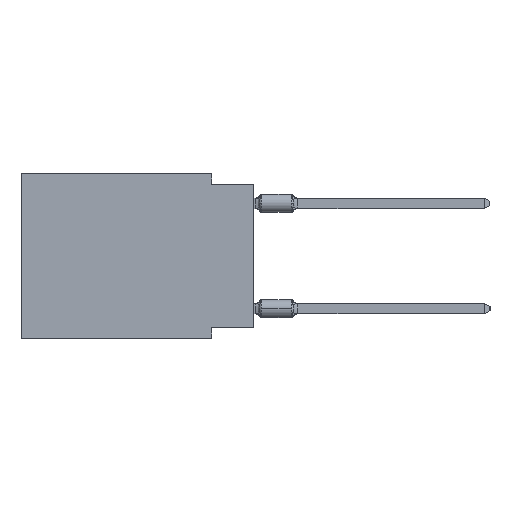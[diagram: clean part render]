
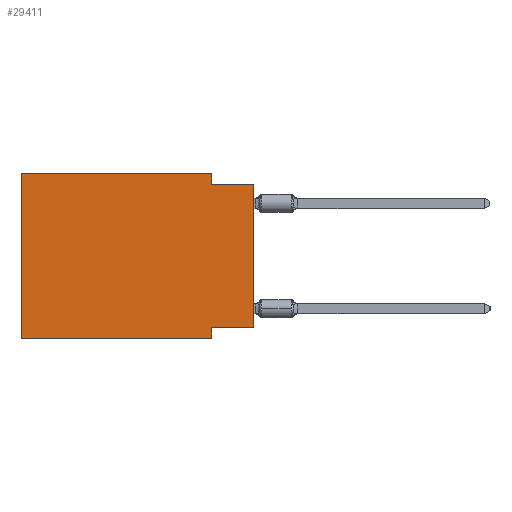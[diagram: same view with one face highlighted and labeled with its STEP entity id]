
A CAD part, left-side view. The second image highlights one B-rep face of the part: STEP entity #29411.
In plain terms, the highlighted planar face has unit normal (-1, 0, 0).
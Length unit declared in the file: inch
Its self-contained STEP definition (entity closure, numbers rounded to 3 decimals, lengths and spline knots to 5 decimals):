
#91 = CARTESIAN_POINT ( 'NONE',  ( 0., 0.1, -0.365 ) ) ;
#154 = ORIENTED_EDGE ( 'NONE', *, *, #16159, .F. ) ;
#680 = CARTESIAN_POINT ( 'NONE',  ( 0., 0.55, 0. ) ) ;
#1687 = EDGE_CURVE ( 'NONE', #15948, #11077, #4665, .T. ) ;
#2459 = EDGE_CURVE ( 'NONE', #29000, #2518, #9080, .T. ) ;
#2518 = VERTEX_POINT ( 'NONE', #11415 ) ;
#3377 = CARTESIAN_POINT ( 'NONE',  ( 0., 0., -0.025 ) ) ;
#4308 = DIRECTION ( 'NONE',  ( 0., 0., -1. ) ) ;
#4665 = LINE ( 'NONE', #29237, #20906 ) ;
#4811 = ORIENTED_EDGE ( 'NONE', *, *, #1687, .T. ) ;
#6917 = VERTEX_POINT ( 'NONE', #23488 ) ;
#7580 = EDGE_CURVE ( 'NONE', #6917, #11077, #14457, .T. ) ;
#8152 = CARTESIAN_POINT ( 'NONE',  ( 0., 0.55, -0.39 ) ) ;
#9080 = LINE ( 'NONE', #680, #9454 ) ;
#9454 = VECTOR ( 'NONE', #25058, 39.37008 ) ;
#10279 = LINE ( 'NONE', #32325, #34799 ) ;
#11077 = VERTEX_POINT ( 'NONE', #31415 ) ;
#11321 = CARTESIAN_POINT ( 'NONE',  ( 0., 0., -0.365 ) ) ;
#11415 = CARTESIAN_POINT ( 'NONE',  ( 0., 0.55, 0. ) ) ;
#11585 = DIRECTION ( 'NONE',  ( 0., -1., 0. ) ) ;
#12739 = DIRECTION ( 'NONE',  ( 0., -1., 0. ) ) ;
#14457 = LINE ( 'NONE', #3377, #26377 ) ;
#14551 = CARTESIAN_POINT ( 'NONE',  ( 0., 0.1, -0.39 ) ) ;
#14753 = CARTESIAN_POINT ( 'NONE',  ( 0., 0.1, 0. ) ) ;
#15461 = EDGE_LOOP ( 'NONE', ( #4811, #27877, #154, #27542, #32997, #31317, #32858, #18688 ) ) ;
#15916 = PLANE ( 'NONE',  #20874 ) ;
#15948 = VERTEX_POINT ( 'NONE', #11321 ) ;
#16159 = EDGE_CURVE ( 'NONE', #31626, #6917, #21309, .T. ) ;
#18160 = CARTESIAN_POINT ( 'NONE',  ( 0., 0.55, -0.39 ) ) ;
#18423 = CARTESIAN_POINT ( 'NONE',  ( 0., 0.55, 0. ) ) ;
#18688 = ORIENTED_EDGE ( 'NONE', *, *, #34823, .F. ) ;
#19564 = EDGE_CURVE ( 'NONE', #29000, #26965, #24652, .T. ) ;
#20874 = AXIS2_PLACEMENT_3D ( 'NONE', #18423, #32076, #26177 ) ;
#20906 = VECTOR ( 'NONE', #34400, 39.37008 ) ;
#21309 = LINE ( 'NONE', #24744, #24211 ) ;
#21341 = LINE ( 'NONE', #21524, #30216 ) ;
#21524 = CARTESIAN_POINT ( 'NONE',  ( 0., 0.55, 0. ) ) ;
#22774 = LINE ( 'NONE', #28706, #32458 ) ;
#22992 = EDGE_CURVE ( 'NONE', #2518, #31626, #21341, .T. ) ;
#23488 = CARTESIAN_POINT ( 'NONE',  ( 0., 0.1, -0.025 ) ) ;
#24211 = VECTOR ( 'NONE', #35107, 39.37008 ) ;
#24272 = DIRECTION ( 'NONE',  ( 0., 1., 0. ) ) ;
#24466 = DIRECTION ( 'NONE',  ( 0., -1., 0. ) ) ;
#24531 = EDGE_CURVE ( 'NONE', #26828, #26965, #22774, .T. ) ;
#24652 = LINE ( 'NONE', #8152, #33983 ) ;
#24744 = CARTESIAN_POINT ( 'NONE',  ( 0., 0.1, 0. ) ) ;
#25058 = DIRECTION ( 'NONE',  ( 0., 0., 1. ) ) ;
#26177 = DIRECTION ( 'NONE',  ( 0., 0., -1. ) ) ;
#26377 = VECTOR ( 'NONE', #11585, 39.37008 ) ;
#26828 = VERTEX_POINT ( 'NONE', #91 ) ;
#26965 = VERTEX_POINT ( 'NONE', #14551 ) ;
#27542 = ORIENTED_EDGE ( 'NONE', *, *, #22992, .F. ) ;
#27877 = ORIENTED_EDGE ( 'NONE', *, *, #7580, .F. ) ;
#28706 = CARTESIAN_POINT ( 'NONE',  ( 0., 0.1, -0.39 ) ) ;
#29000 = VERTEX_POINT ( 'NONE', #18160 ) ;
#29237 = CARTESIAN_POINT ( 'NONE',  ( 0., 0., 0. ) ) ;
#29393 = FACE_OUTER_BOUND ( 'NONE', #15461, .T. ) ;
#29411 = ADVANCED_FACE ( 'NONE', ( #29393 ), #15916, .F. ) ;
#30216 = VECTOR ( 'NONE', #12739, 39.37008 ) ;
#31317 = ORIENTED_EDGE ( 'NONE', *, *, #19564, .T. ) ;
#31415 = CARTESIAN_POINT ( 'NONE',  ( 0., 0., -0.025 ) ) ;
#31626 = VERTEX_POINT ( 'NONE', #14753 ) ;
#32076 = DIRECTION ( 'NONE',  ( 1., 0., 0. ) ) ;
#32325 = CARTESIAN_POINT ( 'NONE',  ( 0., 0., -0.365 ) ) ;
#32458 = VECTOR ( 'NONE', #4308, 39.37008 ) ;
#32858 = ORIENTED_EDGE ( 'NONE', *, *, #24531, .F. ) ;
#32997 = ORIENTED_EDGE ( 'NONE', *, *, #2459, .F. ) ;
#33983 = VECTOR ( 'NONE', #24466, 39.37008 ) ;
#34400 = DIRECTION ( 'NONE',  ( 0., 0., 1. ) ) ;
#34799 = VECTOR ( 'NONE', #24272, 39.37008 ) ;
#34823 = EDGE_CURVE ( 'NONE', #15948, #26828, #10279, .T. ) ;
#35107 = DIRECTION ( 'NONE',  ( 0., 0., -1. ) ) ;
